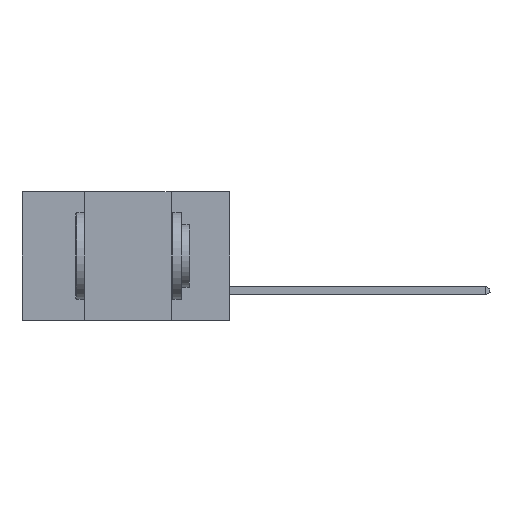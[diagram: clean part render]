
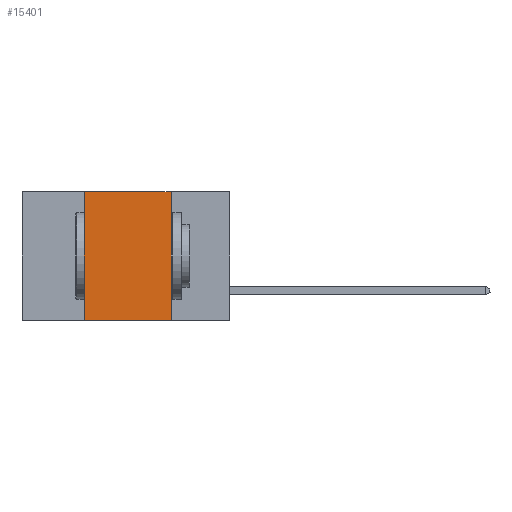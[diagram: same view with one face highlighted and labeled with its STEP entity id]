
A CAD part, left-side view. The second image highlights one B-rep face of the part: STEP entity #15401.
In plain terms, the highlighted planar face has unit normal (-1, 0, 0).
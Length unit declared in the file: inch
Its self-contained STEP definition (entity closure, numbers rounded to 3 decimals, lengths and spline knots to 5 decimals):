
#494 = VECTOR ( 'NONE', #21357, 39.37008 ) ;
#808 = DIRECTION ( 'NONE',  ( 0., -1., 0. ) ) ;
#841 = VERTEX_POINT ( 'NONE', #9613 ) ;
#2293 = LINE ( 'NONE', #15393, #7565 ) ;
#4160 = EDGE_CURVE ( 'NONE', #7747, #8790, #2293, .T. ) ;
#4553 = DIRECTION ( 'NONE',  ( 1., 0., 0. ) ) ;
#4639 = LINE ( 'NONE', #8983, #494 ) ;
#4849 = CARTESIAN_POINT ( 'NONE',  ( 0., 0.42, -0.37 ) ) ;
#6348 = PLANE ( 'NONE',  #22441 ) ;
#6502 = CARTESIAN_POINT ( 'NONE',  ( 0., 0.42, 0. ) ) ;
#6540 = FACE_OUTER_BOUND ( 'NONE', #20208, .T. ) ;
#6583 = DIRECTION ( 'NONE',  ( 0., 0., -1. ) ) ;
#7457 = CARTESIAN_POINT ( 'NONE',  ( 0., 0.6, -0.37 ) ) ;
#7565 = VECTOR ( 'NONE', #12115, 39.37008 ) ;
#7747 = VERTEX_POINT ( 'NONE', #4849 ) ;
#8790 = VERTEX_POINT ( 'NONE', #6502 ) ;
#8936 = EDGE_CURVE ( 'NONE', #7747, #841, #17658, .T. ) ;
#8983 = CARTESIAN_POINT ( 'NONE',  ( 0., 0.6, 0. ) ) ;
#9392 = VECTOR ( 'NONE', #808, 39.37008 ) ;
#9613 = CARTESIAN_POINT ( 'NONE',  ( 0., 0.17, -0.37 ) ) ;
#9997 = EDGE_CURVE ( 'NONE', #8790, #20877, #4639, .T. ) ;
#10664 = CARTESIAN_POINT ( 'NONE',  ( 0., 0.17, 0. ) ) ;
#10914 = CARTESIAN_POINT ( 'NONE',  ( 0., 0.17, 0. ) ) ;
#11631 = CARTESIAN_POINT ( 'NONE',  ( 0., 0.6, 0. ) ) ;
#12115 = DIRECTION ( 'NONE',  ( 0., 0., 1. ) ) ;
#13347 = ORIENTED_EDGE ( 'NONE', *, *, #18190, .F. ) ;
#13998 = LINE ( 'NONE', #10914, #19786 ) ;
#14148 = ORIENTED_EDGE ( 'NONE', *, *, #8936, .T. ) ;
#15393 = CARTESIAN_POINT ( 'NONE',  ( 0., 0.42, 0. ) ) ;
#15401 = ADVANCED_FACE ( 'NONE', ( #6540 ), #6348, .F. ) ;
#15729 = ORIENTED_EDGE ( 'NONE', *, *, #4160, .F. ) ;
#16251 = DIRECTION ( 'NONE',  ( 0., 0., -1. ) ) ;
#17658 = LINE ( 'NONE', #7457, #9392 ) ;
#18190 = EDGE_CURVE ( 'NONE', #20877, #841, #13998, .T. ) ;
#19786 = VECTOR ( 'NONE', #16251, 39.37008 ) ;
#20208 = EDGE_LOOP ( 'NONE', ( #13347, #22307, #15729, #14148 ) ) ;
#20877 = VERTEX_POINT ( 'NONE', #10664 ) ;
#21357 = DIRECTION ( 'NONE',  ( 0., -1., 0. ) ) ;
#22307 = ORIENTED_EDGE ( 'NONE', *, *, #9997, .F. ) ;
#22441 = AXIS2_PLACEMENT_3D ( 'NONE', #11631, #4553, #6583 ) ;
